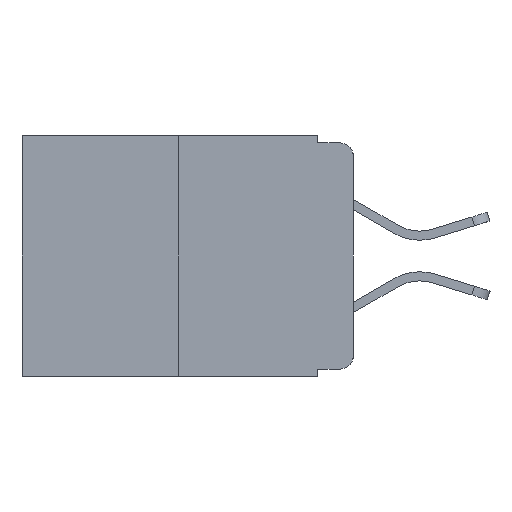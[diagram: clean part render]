
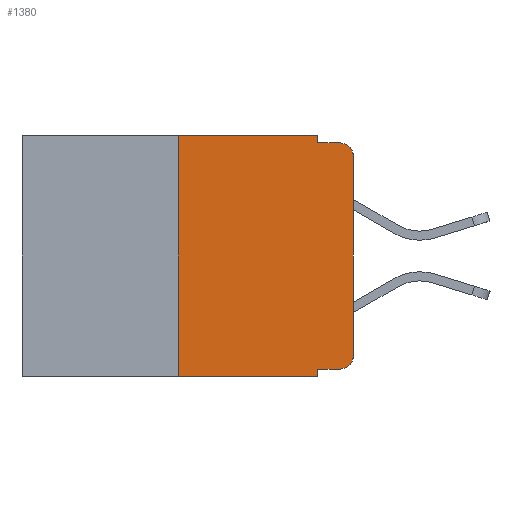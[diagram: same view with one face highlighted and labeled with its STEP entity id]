
A CAD part, left-side view. The second image highlights one B-rep face of the part: STEP entity #1380.
In plain terms, the highlighted planar face has unit normal (-1, 0, 0).
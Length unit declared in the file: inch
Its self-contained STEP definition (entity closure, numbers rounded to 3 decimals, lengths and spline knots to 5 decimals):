
#13 = DIRECTION ( 'NONE',  ( 0., 0., 1. ) ) ;
#414 = DIRECTION ( 'NONE',  ( 0., -1., 0. ) ) ;
#449 = DIRECTION ( 'NONE',  ( 0., 0., -1. ) ) ;
#460 = VERTEX_POINT ( 'NONE', #5894 ) ;
#561 = ORIENTED_EDGE ( 'NONE', *, *, #3637, .T. ) ;
#574 = ORIENTED_EDGE ( 'NONE', *, *, #9136, .F. ) ;
#880 = LINE ( 'NONE', #2293, #9095 ) ;
#881 = EDGE_CURVE ( 'NONE', #460, #3312, #6267, .T. ) ;
#918 = EDGE_CURVE ( 'NONE', #1025, #3312, #4091, .T. ) ;
#1025 = VERTEX_POINT ( 'NONE', #7157 ) ;
#1143 = CARTESIAN_POINT ( 'NONE',  ( 0., 0.051, -0.333 ) ) ;
#1179 = CARTESIAN_POINT ( 'NONE',  ( 0., 0.02, -0.03 ) ) ;
#1217 = DIRECTION ( 'NONE',  ( 0., 0., -1. ) ) ;
#1222 = ORIENTED_EDGE ( 'NONE', *, *, #1993, .F. ) ;
#1238 = VECTOR ( 'NONE', #8613, 39.37008 ) ;
#1243 = AXIS2_PLACEMENT_3D ( 'NONE', #1179, #4226, #1217 ) ;
#1264 = CARTESIAN_POINT ( 'NONE',  ( 0., 0.473, 0. ) ) ;
#1380 = ADVANCED_FACE ( 'NONE', ( #9679 ), #9728, .F. ) ;
#1537 = DIRECTION ( 'NONE',  ( 0., 0., -1. ) ) ;
#1578 = LINE ( 'NONE', #1264, #9853 ) ;
#1858 = LINE ( 'NONE', #9543, #9571 ) ;
#1993 = EDGE_CURVE ( 'NONE', #4007, #2113, #7664, .T. ) ;
#2006 = DIRECTION ( 'NONE',  ( 0., 0., 1. ) ) ;
#2069 = CARTESIAN_POINT ( 'NONE',  ( 0., 0.051, 0. ) ) ;
#2113 = VERTEX_POINT ( 'NONE', #3286 ) ;
#2171 = EDGE_CURVE ( 'NONE', #1025, #7070, #8559, .T. ) ;
#2192 = VERTEX_POINT ( 'NONE', #9478 ) ;
#2237 = ORIENTED_EDGE ( 'NONE', *, *, #881, .T. ) ;
#2293 = CARTESIAN_POINT ( 'NONE',  ( 0., 0.25, 0. ) ) ;
#2531 = CARTESIAN_POINT ( 'NONE',  ( 0., 0.051, 0. ) ) ;
#2730 = EDGE_CURVE ( 'NONE', #8186, #2192, #5549, .T. ) ;
#2903 = CARTESIAN_POINT ( 'NONE',  ( 0., 0.473, 0. ) ) ;
#3286 = CARTESIAN_POINT ( 'NONE',  ( 0., 0.051, -0.01 ) ) ;
#3312 = VERTEX_POINT ( 'NONE', #5441 ) ;
#3455 = CARTESIAN_POINT ( 'NONE',  ( 0., 0.051, -0.01 ) ) ;
#3541 = CARTESIAN_POINT ( 'NONE',  ( 0., 0.02, -0.313 ) ) ;
#3637 = EDGE_CURVE ( 'NONE', #7070, #6729, #6383, .T. ) ;
#3845 = AXIS2_PLACEMENT_3D ( 'NONE', #3541, #6555, #5817 ) ;
#3934 = CARTESIAN_POINT ( 'NONE',  ( 0., 0.473, -0.343 ) ) ;
#4007 = VERTEX_POINT ( 'NONE', #2069 ) ;
#4041 = ORIENTED_EDGE ( 'NONE', *, *, #5879, .F. ) ;
#4091 = LINE ( 'NONE', #2531, #4764 ) ;
#4226 = DIRECTION ( 'NONE',  ( -1., 0., 0. ) ) ;
#4256 = CARTESIAN_POINT ( 'NONE',  ( 0., 0., -0.03 ) ) ;
#4764 = VECTOR ( 'NONE', #6943, 39.37008 ) ;
#5338 = CARTESIAN_POINT ( 'NONE',  ( 0., 0.051, 0. ) ) ;
#5441 = CARTESIAN_POINT ( 'NONE',  ( 0., 0.051, -0.343 ) ) ;
#5549 = CIRCLE ( 'NONE', #1243, 0.02 ) ;
#5693 = DIRECTION ( 'NONE',  ( 0., -1., 0. ) ) ;
#5805 = CARTESIAN_POINT ( 'NONE',  ( 0., 0.25, 0. ) ) ;
#5817 = DIRECTION ( 'NONE',  ( 0., 0., -1. ) ) ;
#5879 = EDGE_CURVE ( 'NONE', #5972, #4007, #1578, .T. ) ;
#5894 = CARTESIAN_POINT ( 'NONE',  ( 0., 0.25, -0.343 ) ) ;
#5972 = VERTEX_POINT ( 'NONE', #5805 ) ;
#6101 = ORIENTED_EDGE ( 'NONE', *, *, #2171, .T. ) ;
#6254 = ORIENTED_EDGE ( 'NONE', *, *, #2730, .T. ) ;
#6262 = CARTESIAN_POINT ( 'NONE',  ( 0., 0.02, -0.333 ) ) ;
#6267 = LINE ( 'NONE', #3934, #1238 ) ;
#6383 = CIRCLE ( 'NONE', #3845, 0.02 ) ;
#6555 = DIRECTION ( 'NONE',  ( -1., 0., 0. ) ) ;
#6698 = AXIS2_PLACEMENT_3D ( 'NONE', #2903, #7334, #449 ) ;
#6729 = VERTEX_POINT ( 'NONE', #9479 ) ;
#6943 = DIRECTION ( 'NONE',  ( 0., 0., -1. ) ) ;
#7070 = VERTEX_POINT ( 'NONE', #6262 ) ;
#7157 = CARTESIAN_POINT ( 'NONE',  ( 0., 0.051, -0.333 ) ) ;
#7334 = DIRECTION ( 'NONE',  ( 1., 0., 0. ) ) ;
#7664 = LINE ( 'NONE', #5338, #8861 ) ;
#7677 = EDGE_LOOP ( 'NONE', ( #9409, #6254, #7809, #1222, #4041, #574, #2237, #8656, #6101, #561 ) ) ;
#7809 = ORIENTED_EDGE ( 'NONE', *, *, #8129, .F. ) ;
#8129 = EDGE_CURVE ( 'NONE', #2113, #2192, #9579, .T. ) ;
#8153 = DIRECTION ( 'NONE',  ( 0., -1., 0. ) ) ;
#8186 = VERTEX_POINT ( 'NONE', #4256 ) ;
#8559 = LINE ( 'NONE', #1143, #9672 ) ;
#8583 = VECTOR ( 'NONE', #5693, 39.37008 ) ;
#8613 = DIRECTION ( 'NONE',  ( 0., -1., 0. ) ) ;
#8656 = ORIENTED_EDGE ( 'NONE', *, *, #918, .F. ) ;
#8861 = VECTOR ( 'NONE', #1537, 39.37008 ) ;
#9095 = VECTOR ( 'NONE', #13, 39.37008 ) ;
#9136 = EDGE_CURVE ( 'NONE', #460, #5972, #880, .T. ) ;
#9409 = ORIENTED_EDGE ( 'NONE', *, *, #9725, .T. ) ;
#9478 = CARTESIAN_POINT ( 'NONE',  ( 0., 0.02, -0.01 ) ) ;
#9479 = CARTESIAN_POINT ( 'NONE',  ( 0., 0., -0.313 ) ) ;
#9543 = CARTESIAN_POINT ( 'NONE',  ( 0., 0., 0. ) ) ;
#9571 = VECTOR ( 'NONE', #2006, 39.37008 ) ;
#9579 = LINE ( 'NONE', #3455, #8583 ) ;
#9672 = VECTOR ( 'NONE', #8153, 39.37008 ) ;
#9679 = FACE_OUTER_BOUND ( 'NONE', #7677, .T. ) ;
#9725 = EDGE_CURVE ( 'NONE', #6729, #8186, #1858, .T. ) ;
#9728 = PLANE ( 'NONE',  #6698 ) ;
#9853 = VECTOR ( 'NONE', #414, 39.37008 ) ;
